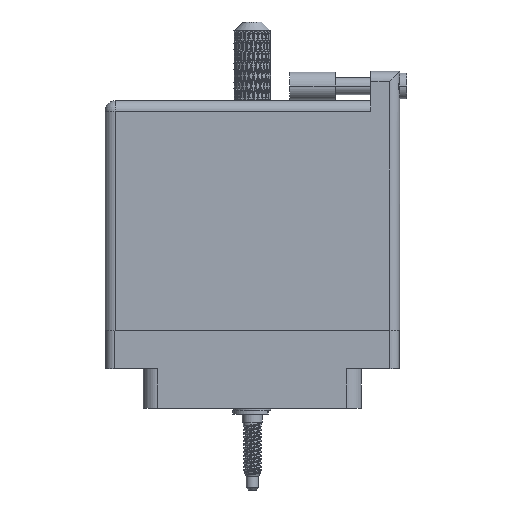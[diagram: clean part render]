
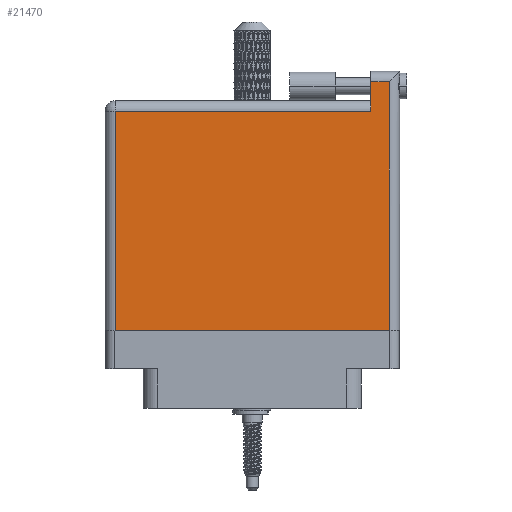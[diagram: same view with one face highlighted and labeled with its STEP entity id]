
A CAD part, front view. The second image highlights one B-rep face of the part: STEP entity #21470.
In plain terms, the highlighted face is planar.
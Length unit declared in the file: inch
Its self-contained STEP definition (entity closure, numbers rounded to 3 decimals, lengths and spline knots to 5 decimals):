
#2263 = CARTESIAN_POINT ( 'NONE',  ( 0., 1.566, 0. ) ) ;
#3430 = LINE ( 'NONE', #51950, #79091 ) ;
#3877 = EDGE_CURVE ( 'NONE', #29351, #70172, #69206, .T. ) ;
#7535 = DIRECTION ( 'NONE',  ( 1., 0., 0. ) ) ;
#7695 = ORIENTED_EDGE ( 'NONE', *, *, #43584, .T. ) ;
#8295 = CARTESIAN_POINT ( 'NONE',  ( 1.811, 1.696, 0. ) ) ;
#10490 = VECTOR ( 'NONE', #75093, 39.37008 ) ;
#11592 = CARTESIAN_POINT ( 'NONE',  ( 0.07, 0., 0. ) ) ;
#13982 = ORIENTED_EDGE ( 'NONE', *, *, #3877, .T. ) ;
#14430 = LINE ( 'NONE', #47728, #101424 ) ;
#15114 = ORIENTED_EDGE ( 'NONE', *, *, #21835, .T. ) ;
#16156 = VERTEX_POINT ( 'NONE', #89607 ) ;
#18709 = CARTESIAN_POINT ( 'NONE',  ( 0.07, 1.496, 0. ) ) ;
#21470 = ADVANCED_FACE ( 'NONE', ( #44799 ), #75458, .F. ) ;
#21835 = EDGE_CURVE ( 'NONE', #16156, #31351, #14430, .T. ) ;
#24581 = ORIENTED_EDGE ( 'NONE', *, *, #67815, .T. ) ;
#27931 = DIRECTION ( 'NONE',  ( -1., 0., 0. ) ) ;
#28402 = ORIENTED_EDGE ( 'NONE', *, *, #87985, .T. ) ;
#29351 = VERTEX_POINT ( 'NONE', #8295 ) ;
#30139 = CARTESIAN_POINT ( 'NONE',  ( 1.938, 1.766, 0. ) ) ;
#31351 = VERTEX_POINT ( 'NONE', #75348 ) ;
#32310 = AXIS2_PLACEMENT_3D ( 'NONE', #2263, #99197, #27931 ) ;
#32435 = EDGE_CURVE ( 'NONE', #31351, #94908, #54176, .T. ) ;
#37039 = LINE ( 'NONE', #83642, #10490 ) ;
#43584 = EDGE_CURVE ( 'NONE', #70172, #43844, #3430, .T. ) ;
#43844 = VERTEX_POINT ( 'NONE', #18709 ) ;
#44799 = FACE_OUTER_BOUND ( 'NONE', #103585, .T. ) ;
#45946 = VECTOR ( 'NONE', #51422, 39.37008 ) ;
#47728 = CARTESIAN_POINT ( 'NONE',  ( 0., 0., 0. ) ) ;
#51422 = DIRECTION ( 'NONE',  ( 0., -1., 0. ) ) ;
#51950 = CARTESIAN_POINT ( 'NONE',  ( 0., 1.496, 0. ) ) ;
#54176 = LINE ( 'NONE', #30139, #65430 ) ;
#55444 = VECTOR ( 'NONE', #61939, 39.37008 ) ;
#60792 = DIRECTION ( 'NONE',  ( -1., 0., 0. ) ) ;
#61939 = DIRECTION ( 'NONE',  ( 0., -1., 0. ) ) ;
#65430 = VECTOR ( 'NONE', #86566, 39.37008 ) ;
#67815 = EDGE_CURVE ( 'NONE', #43844, #16156, #79985, .T. ) ;
#69206 = LINE ( 'NONE', #77020, #55444 ) ;
#70172 = VERTEX_POINT ( 'NONE', #79353 ) ;
#75093 = DIRECTION ( 'NONE',  ( -1., 0., 0. ) ) ;
#75348 = CARTESIAN_POINT ( 'NONE',  ( 1.938, 0., 0. ) ) ;
#75458 = PLANE ( 'NONE',  #32310 ) ;
#77020 = CARTESIAN_POINT ( 'NONE',  ( 1.811, 1.766, 0. ) ) ;
#79091 = VECTOR ( 'NONE', #60792, 39.37008 ) ;
#79353 = CARTESIAN_POINT ( 'NONE',  ( 1.811, 1.496, 0. ) ) ;
#79985 = LINE ( 'NONE', #11592, #45946 ) ;
#83642 = CARTESIAN_POINT ( 'NONE',  ( 0., 1.696, 0. ) ) ;
#84430 = ORIENTED_EDGE ( 'NONE', *, *, #32435, .T. ) ;
#86566 = DIRECTION ( 'NONE',  ( 0., 1., 0. ) ) ;
#87985 = EDGE_CURVE ( 'NONE', #94908, #29351, #37039, .T. ) ;
#89607 = CARTESIAN_POINT ( 'NONE',  ( 0.07, 0., 0. ) ) ;
#94908 = VERTEX_POINT ( 'NONE', #103749 ) ;
#99197 = DIRECTION ( 'NONE',  ( 0., 0., -1. ) ) ;
#101424 = VECTOR ( 'NONE', #7535, 39.37008 ) ;
#103585 = EDGE_LOOP ( 'NONE', ( #15114, #84430, #28402, #13982, #7695, #24581 ) ) ;
#103749 = CARTESIAN_POINT ( 'NONE',  ( 1.938, 1.696, 0. ) ) ;
